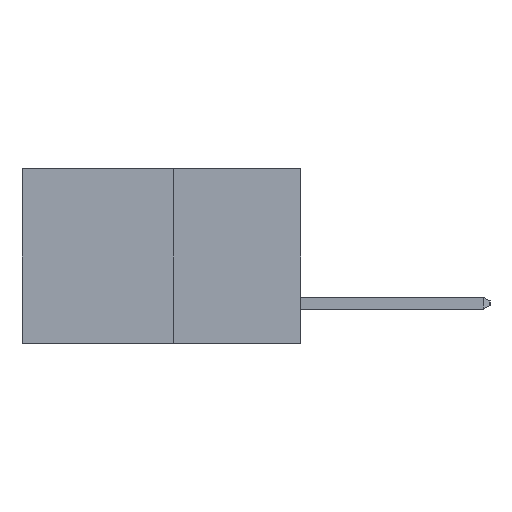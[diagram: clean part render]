
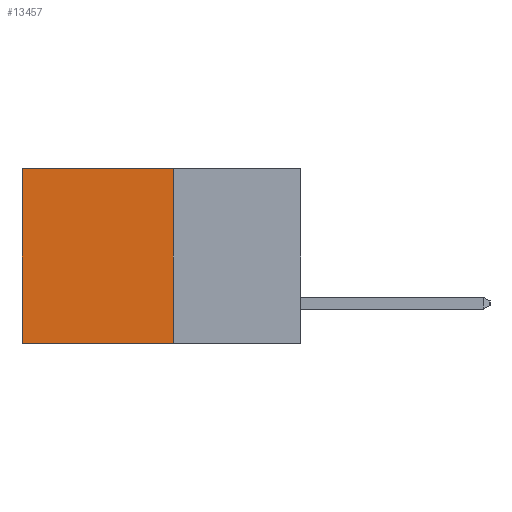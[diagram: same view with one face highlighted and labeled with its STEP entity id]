
A CAD part, left-side view. The second image highlights one B-rep face of the part: STEP entity #13457.
In plain terms, the highlighted planar face has unit normal (-1, 0, 0).
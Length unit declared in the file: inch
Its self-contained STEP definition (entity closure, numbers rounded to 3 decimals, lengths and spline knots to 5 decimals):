
#3 = ORIENTED_EDGE ( 'NONE', *, *, #388, .F. ) ;
#388 = EDGE_CURVE ( 'NONE', #5583, #8082, #11131, .T. ) ;
#553 = EDGE_LOOP ( 'NONE', ( #14286, #14633, #3, #4119 ) ) ;
#856 = EDGE_CURVE ( 'NONE', #5583, #13869, #7867, .T. ) ;
#1026 = EDGE_CURVE ( 'NONE', #8082, #5068, #14440, .T. ) ;
#2274 = CARTESIAN_POINT ( 'NONE',  ( 0.277, 0.27, -0.37 ) ) ;
#2444 = DIRECTION ( 'NONE',  ( 0., 0., -1. ) ) ;
#2833 = CARTESIAN_POINT ( 'NONE',  ( 0.277, 0.27, -0.37 ) ) ;
#4119 = ORIENTED_EDGE ( 'NONE', *, *, #856, .T. ) ;
#4924 = CARTESIAN_POINT ( 'NONE',  ( 0.277, 0.59, -0.37 ) ) ;
#5023 = VECTOR ( 'NONE', #12677, 39.37008 ) ;
#5068 = VERTEX_POINT ( 'NONE', #14126 ) ;
#5325 = DIRECTION ( 'NONE',  ( 0., 1., 0. ) ) ;
#5583 = VERTEX_POINT ( 'NONE', #8229 ) ;
#5708 = AXIS2_PLACEMENT_3D ( 'NONE', #2274, #14420, #7191 ) ;
#6438 = LINE ( 'NONE', #4924, #9679 ) ;
#6968 = CARTESIAN_POINT ( 'NONE',  ( 0.277, 0.59, 0. ) ) ;
#7191 = DIRECTION ( 'NONE',  ( 0., 0., -1. ) ) ;
#7867 = LINE ( 'NONE', #12107, #5023 ) ;
#8082 = VERTEX_POINT ( 'NONE', #8710 ) ;
#8229 = CARTESIAN_POINT ( 'NONE',  ( 0.277, 0.27, 0. ) ) ;
#8710 = CARTESIAN_POINT ( 'NONE',  ( 0.277, 0.27, -0.37 ) ) ;
#9679 = VECTOR ( 'NONE', #2444, 39.37008 ) ;
#11131 = LINE ( 'NONE', #13275, #13906 ) ;
#11300 = VECTOR ( 'NONE', #5325, 39.37008 ) ;
#12107 = CARTESIAN_POINT ( 'NONE',  ( 0.277, 0.27, 0. ) ) ;
#12677 = DIRECTION ( 'NONE',  ( 0., 1., 0. ) ) ;
#12713 = DIRECTION ( 'NONE',  ( 0., 0., -1. ) ) ;
#12941 = FACE_OUTER_BOUND ( 'NONE', #553, .T. ) ;
#13257 = PLANE ( 'NONE',  #5708 ) ;
#13275 = CARTESIAN_POINT ( 'NONE',  ( 0.277, 0.27, -0.37 ) ) ;
#13457 = ADVANCED_FACE ( 'NONE', ( #12941 ), #13257, .F. ) ;
#13869 = VERTEX_POINT ( 'NONE', #6968 ) ;
#13906 = VECTOR ( 'NONE', #12713, 39.37008 ) ;
#14126 = CARTESIAN_POINT ( 'NONE',  ( 0.277, 0.59, -0.37 ) ) ;
#14286 = ORIENTED_EDGE ( 'NONE', *, *, #15351, .T. ) ;
#14420 = DIRECTION ( 'NONE',  ( 1., 0., 0. ) ) ;
#14440 = LINE ( 'NONE', #2833, #11300 ) ;
#14633 = ORIENTED_EDGE ( 'NONE', *, *, #1026, .F. ) ;
#15351 = EDGE_CURVE ( 'NONE', #13869, #5068, #6438, .T. ) ;
